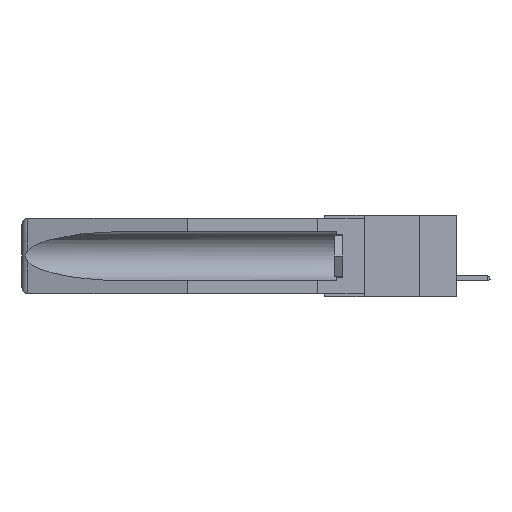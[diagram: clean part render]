
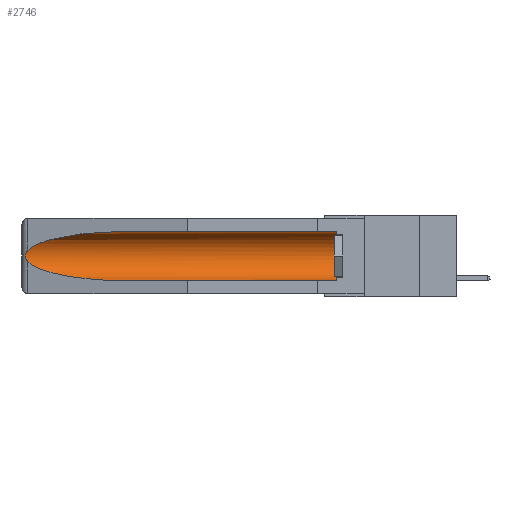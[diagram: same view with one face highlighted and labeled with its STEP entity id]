
A CAD part, left-side view. The second image highlights one B-rep face of the part: STEP entity #2746.
In plain terms, the highlighted cylindrical face has radius 2.857 mm (diameter 5.715 mm), a partial arc.
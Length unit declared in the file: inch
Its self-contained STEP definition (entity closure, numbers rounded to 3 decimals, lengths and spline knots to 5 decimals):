
#278 = EDGE_CURVE ( 'NONE', #6411, #11983, #10132, .T. ) ;
#364 = CARTESIAN_POINT ( 'NONE',  ( 0.21114, 1.30732, -0.059 ) ) ;
#585 = CARTESIAN_POINT ( 'NONE',  ( 0.26597, 1.5296, -0.19026 ) ) ;
#2281 = LINE ( 'NONE', #11156, #21733 ) ;
#2746 = ADVANCED_FACE ( 'NONE', ( #19872 ), #17619, .F. ) ;
#3109 = LINE ( 'NONE', #16988, #12462 ) ;
#3383 = CARTESIAN_POINT ( 'NONE',  ( 0.155, 1.07973, -0.059 ) ) ;
#3778 = CARTESIAN_POINT ( 'NONE',  ( 0.155, 1.07973, -0.059 ) ) ;
#3987 = CARTESIAN_POINT ( 'NONE',  ( 0.26537, 1.52718, -0.19328 ) ) ;
#4875 = ORIENTED_EDGE ( 'NONE', *, *, #15928, .T. ) ;
#5137 = VERTEX_POINT ( 'NONE', #3383 ) ;
#5685 = DIRECTION ( 'NONE',  ( 0., -1., 0. ) ) ;
#5827 = CARTESIAN_POINT ( 'NONE',  ( 0.26537, 1.52718, -0.14972 ) ) ;
#6411 = VERTEX_POINT ( 'NONE', #6539 ) ;
#6539 = CARTESIAN_POINT ( 'NONE',  ( 0.155, 0.126, -0.284 ) ) ;
#6974 = CARTESIAN_POINT ( 'NONE',  ( 0.26537, 1.52718, -0.19328 ) ) ;
#7417 = CARTESIAN_POINT ( 'NONE',  ( 0.25451, 1.48313, -0.09465 ) ) ;
#8091 = EDGE_CURVE ( 'NONE', #5137, #19115, #18750, .T. ) ;
#8103 = DIRECTION ( 'NONE',  ( 0., 1., 0. ) ) ;
#8362 = B_SPLINE_CURVE_WITH_KNOTS ( 'NONE', 3,
 ( #13225, #16681, #18351, #22049, #11418, #16454, #20261, #9450, #585, #3987 ),
 .UNSPECIFIED., .F., .F.,
 ( 4, 2, 2, 2, 4 ),
 ( 0., 0.00029, 0.00058, 0.00087, 0.00117 ),
 .UNSPECIFIED. ) ;
#8853 = EDGE_CURVE ( 'NONE', #20252, #10997, #15293, .T. ) ;
#8896 = EDGE_CURVE ( 'NONE', #11983, #5137, #2281, .T. ) ;
#9042 = DIRECTION ( 'NONE',  ( 0., 0., 1. ) ) ;
#9268 = CARTESIAN_POINT ( 'NONE',  ( 0.25451, 1.48313, -0.24835 ) ) ;
#9450 = CARTESIAN_POINT ( 'NONE',  ( 0.26655, 1.53094, -0.18657 ) ) ;
#9807 = DIRECTION ( 'NONE',  ( 0., 1., 0. ) ) ;
#10132 = CIRCLE ( 'NONE', #16118, 0.1125 ) ;
#10857 = EDGE_LOOP ( 'NONE', ( #12693, #4875, #12756, #19547, #13885, #13349 ) ) ;
#10958 = CARTESIAN_POINT ( 'NONE',  ( 0.26537, 1.52718, -0.14972 ) ) ;
#10997 = VERTEX_POINT ( 'NONE', #13348 ) ;
#11076 = CARTESIAN_POINT ( 'NONE',  ( 0.21114, 1.30732, -0.284 ) ) ;
#11156 = CARTESIAN_POINT ( 'NONE',  ( 0.155, -0.30754, -0.059 ) ) ;
#11418 = CARTESIAN_POINT ( 'NONE',  ( 0.2675, 1.53308, -0.16763 ) ) ;
#11983 = VERTEX_POINT ( 'NONE', #20249 ) ;
#12462 = VECTOR ( 'NONE', #8103, 39.37008 ) ;
#12693 = ORIENTED_EDGE ( 'NONE', *, *, #8091, .T. ) ;
#12716 = CARTESIAN_POINT ( 'NONE',  ( 0.155, 0.126, -0.1715 ) ) ;
#12756 = ORIENTED_EDGE ( 'NONE', *, *, #8853, .T. ) ;
#13225 = CARTESIAN_POINT ( 'NONE',  ( 0.26537, 1.52718, -0.14972 ) ) ;
#13348 = CARTESIAN_POINT ( 'NONE',  ( 0.155, 1.07973, -0.284 ) ) ;
#13349 = ORIENTED_EDGE ( 'NONE', *, *, #8896, .T. ) ;
#13885 = ORIENTED_EDGE ( 'NONE', *, *, #278, .T. ) ;
#14336 = CARTESIAN_POINT ( 'NONE',  ( 0.155, 1.07973, -0.284 ) ) ;
#15293 =( BOUNDED_CURVE ( )  B_SPLINE_CURVE ( 3, ( #19984, #9268, #11076, #14336 ),
 .UNSPECIFIED., .F., .F. ) 
 B_SPLINE_CURVE_WITH_KNOTS ( ( 4, 4 ),
 ( 0.1948, 1.5708 ),
 .UNSPECIFIED. ) 
 CURVE ( )  GEOMETRIC_REPRESENTATION_ITEM ( )  RATIONAL_B_SPLINE_CURVE ( ( 1., 0.848, 0.848, 1. ) ) 
 REPRESENTATION_ITEM ( '' )  );
#15928 = EDGE_CURVE ( 'NONE', #19115, #20252, #8362, .T. ) ;
#16029 = EDGE_CURVE ( 'NONE', #6411, #10997, #3109, .T. ) ;
#16118 = AXIS2_PLACEMENT_3D ( 'NONE', #12716, #5685, #18460 ) ;
#16300 = CARTESIAN_POINT ( 'NONE',  ( 0.155, -0.30754, -0.1715 ) ) ;
#16454 = CARTESIAN_POINT ( 'NONE',  ( 0.2675, 1.53308, -0.17534 ) ) ;
#16681 = CARTESIAN_POINT ( 'NONE',  ( 0.26597, 1.52961, -0.15275 ) ) ;
#16988 = CARTESIAN_POINT ( 'NONE',  ( 0.155, -0.30754, -0.284 ) ) ;
#17619 = CYLINDRICAL_SURFACE ( 'NONE', #20088, 0.1125 ) ;
#18100 = DIRECTION ( 'NONE',  ( 0., 1., 0. ) ) ;
#18351 = CARTESIAN_POINT ( 'NONE',  ( 0.26654, 1.53092, -0.15636 ) ) ;
#18460 = DIRECTION ( 'NONE',  ( 0., 0., 1. ) ) ;
#18750 =( BOUNDED_CURVE ( )  B_SPLINE_CURVE ( 3, ( #3778, #364, #7417, #5827 ),
 .UNSPECIFIED., .F., .T. ) 
 B_SPLINE_CURVE_WITH_KNOTS ( ( 4, 4 ),
 ( 4.71239, 6.08839 ),
 .UNSPECIFIED. ) 
 CURVE ( )  GEOMETRIC_REPRESENTATION_ITEM ( )  RATIONAL_B_SPLINE_CURVE ( ( 1., 0.848, 0.848, 1. ) ) 
 REPRESENTATION_ITEM ( '' )  );
#19115 = VERTEX_POINT ( 'NONE', #10958 ) ;
#19547 = ORIENTED_EDGE ( 'NONE', *, *, #16029, .F. ) ;
#19872 = FACE_OUTER_BOUND ( 'NONE', #10857, .T. ) ;
#19984 = CARTESIAN_POINT ( 'NONE',  ( 0.26537, 1.52718, -0.19328 ) ) ;
#20088 = AXIS2_PLACEMENT_3D ( 'NONE', #16300, #18100, #9042 ) ;
#20249 = CARTESIAN_POINT ( 'NONE',  ( 0.155, 0.126, -0.059 ) ) ;
#20252 = VERTEX_POINT ( 'NONE', #6974 ) ;
#20261 = CARTESIAN_POINT ( 'NONE',  ( 0.2673, 1.53269, -0.17917 ) ) ;
#21733 = VECTOR ( 'NONE', #9807, 39.37008 ) ;
#22049 = CARTESIAN_POINT ( 'NONE',  ( 0.2673, 1.5327, -0.16383 ) ) ;
